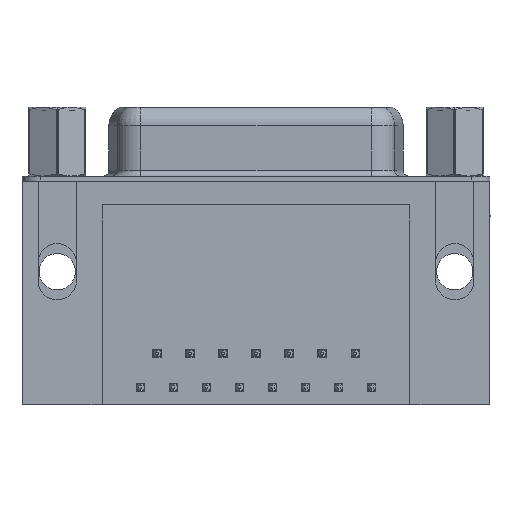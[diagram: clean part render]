
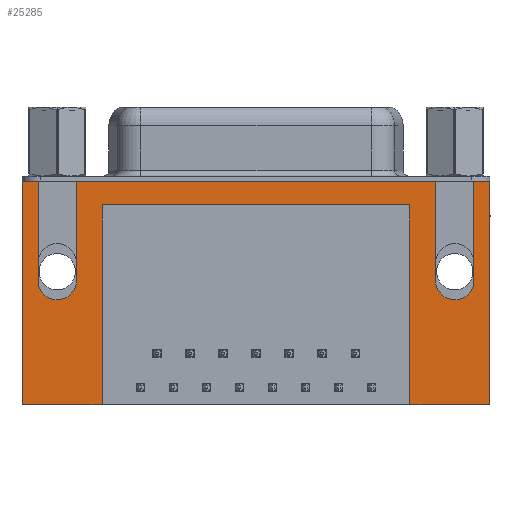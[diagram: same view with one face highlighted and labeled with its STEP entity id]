
A CAD part, front view. The second image highlights one B-rep face of the part: STEP entity #25285.
In plain terms, the highlighted planar face has unit normal (0, -1, 0).
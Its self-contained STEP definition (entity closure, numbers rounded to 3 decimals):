
#57 = EDGE_CURVE ( 'NONE', #28058, #2668, #22435, .T. ) ;
#464 = EDGE_CURVE ( 'NONE', #23235, #28058, #17280, .T. ) ;
#732 = FACE_OUTER_BOUND ( 'NONE', #28871, .T. ) ;
#1025 = EDGE_CURVE ( 'NONE', #8526, #19001, #14842, .T. ) ;
#1231 = DIRECTION ( 'NONE',  ( -1., 0., 0. ) ) ;
#1499 = LINE ( 'NONE', #9939, #1564 ) ;
#1564 = VECTOR ( 'NONE', #26962, 1000. ) ;
#1758 = CARTESIAN_POINT ( 'NONE',  ( 31.72, -6.275, 0. ) ) ;
#1853 = CARTESIAN_POINT ( 'NONE',  ( -2.935, -6.275, -2.5 ) ) ;
#2569 = VECTOR ( 'NONE', #21435, 1000. ) ;
#2662 = LINE ( 'NONE', #19008, #2569 ) ;
#2668 = VERTEX_POINT ( 'NONE', #8424 ) ;
#4235 = DIRECTION ( 'NONE',  ( 0., 0., 1. ) ) ;
#4272 = VERTEX_POINT ( 'NONE', #16402 ) ;
#4550 = DIRECTION ( 'NONE',  ( 0., 0., 1. ) ) ;
#4553 = VECTOR ( 'NONE', #14404, 1000. ) ;
#4650 = AXIS2_PLACEMENT_3D ( 'NONE', #19683, #5103, #22114 ) ;
#4806 = DIRECTION ( 'NONE',  ( 0., 0., -1. ) ) ;
#4980 = LINE ( 'NONE', #9600, #4553 ) ;
#5020 = ORIENTED_EDGE ( 'NONE', *, *, #29779, .F. ) ;
#5103 = DIRECTION ( 'NONE',  ( 0., -1., 0. ) ) ;
#5549 = VERTEX_POINT ( 'NONE', #13573 ) ;
#5914 = VERTEX_POINT ( 'NONE', #16620 ) ;
#6370 = CARTESIAN_POINT ( 'NONE',  ( 34.92, -6.275, 0. ) ) ;
#6408 = CARTESIAN_POINT ( 'NONE',  ( -2.935, -6.275, 0. ) ) ;
#6509 = DIRECTION ( 'NONE',  ( 0., -1., 0. ) ) ;
#6653 = CARTESIAN_POINT ( 'NONE',  ( -1.6, -6.275, 0. ) ) ;
#6703 = VERTEX_POINT ( 'NONE', #22931 ) ;
#6790 = ORIENTED_EDGE ( 'NONE', *, *, #464, .F. ) ;
#6910 = CARTESIAN_POINT ( 'NONE',  ( 36.255, -6.275, -18.76 ) ) ;
#7192 = VECTOR ( 'NONE', #26026, 1000. ) ;
#7223 = ORIENTED_EDGE ( 'NONE', *, *, #26447, .F. ) ;
#7283 = ORIENTED_EDGE ( 'NONE', *, *, #20444, .F. ) ;
#7373 = EDGE_CURVE ( 'NONE', #11342, #30143, #14511, .T. ) ;
#7556 = LINE ( 'NONE', #6408, #7192 ) ;
#8424 = CARTESIAN_POINT ( 'NONE',  ( 29.555, -6.275, -2. ) ) ;
#8526 = VERTEX_POINT ( 'NONE', #12347 ) ;
#8750 = CARTESIAN_POINT ( 'NONE',  ( 34.92, -6.275, 0. ) ) ;
#8834 = EDGE_CURVE ( 'NONE', #17516, #10612, #7556, .T. ) ;
#9586 = CARTESIAN_POINT ( 'NONE',  ( 36.255, -6.275, 0. ) ) ;
#9600 = CARTESIAN_POINT ( 'NONE',  ( 36.255, -6.275, -18.76 ) ) ;
#9855 = VECTOR ( 'NONE', #26143, 1000. ) ;
#9884 = LINE ( 'NONE', #6653, #9855 ) ;
#9939 = CARTESIAN_POINT ( 'NONE',  ( 31.72, -6.275, 0. ) ) ;
#10142 = EDGE_CURVE ( 'NONE', #19001, #5549, #1499, .T. ) ;
#10612 = VERTEX_POINT ( 'NONE', #9586 ) ;
#10784 = AXIS2_PLACEMENT_3D ( 'NONE', #24204, #19395, #4806 ) ;
#10906 = LINE ( 'NONE', #6370, #10937 ) ;
#10937 = VECTOR ( 'NONE', #23394, 1000. ) ;
#10995 = CARTESIAN_POINT ( 'NONE',  ( 3.765, -6.275, -2. ) ) ;
#11342 = VERTEX_POINT ( 'NONE', #25682 ) ;
#11384 = DIRECTION ( 'NONE',  ( -1., 0., 0. ) ) ;
#12347 = CARTESIAN_POINT ( 'NONE',  ( 1.6, -6.275, 0. ) ) ;
#12406 = EDGE_CURVE ( 'NONE', #6703, #24073, #23464, .T. ) ;
#13284 = DIRECTION ( 'NONE',  ( 1., 0., 0. ) ) ;
#13573 = CARTESIAN_POINT ( 'NONE',  ( 31.72, -6.275, -8.35 ) ) ;
#14277 = VECTOR ( 'NONE', #13284, 1000. ) ;
#14365 = ORIENTED_EDGE ( 'NONE', *, *, #24618, .T. ) ;
#14404 = DIRECTION ( 'NONE',  ( -1., 0., 0. ) ) ;
#14511 = CIRCLE ( 'NONE', #26122, 1.6 ) ;
#14842 = LINE ( 'NONE', #17664, #14927 ) ;
#14927 = VECTOR ( 'NONE', #28921, 1000. ) ;
#14974 = LINE ( 'NONE', #15721, #14277 ) ;
#15721 = CARTESIAN_POINT ( 'NONE',  ( -2.935, -6.275, 0. ) ) ;
#16050 = EDGE_CURVE ( 'NONE', #2668, #6703, #30447, .T. ) ;
#16227 = CARTESIAN_POINT ( 'NONE',  ( 29.555, -6.275, -2. ) ) ;
#16236 = ORIENTED_EDGE ( 'NONE', *, *, #18652, .F. ) ;
#16402 = CARTESIAN_POINT ( 'NONE',  ( -1.6, -6.275, 0. ) ) ;
#16620 = CARTESIAN_POINT ( 'NONE',  ( -2.935, -6.275, -18.76 ) ) ;
#16688 = VERTEX_POINT ( 'NONE', #18237 ) ;
#16695 = ORIENTED_EDGE ( 'NONE', *, *, #19280, .F. ) ;
#16969 = PLANE ( 'NONE',  #10784 ) ;
#17258 = CARTESIAN_POINT ( 'NONE',  ( 1.6, -6.275, -8.35 ) ) ;
#17280 = LINE ( 'NONE', #6910, #17444 ) ;
#17444 = VECTOR ( 'NONE', #11384, 1000. ) ;
#17516 = VERTEX_POINT ( 'NONE', #8750 ) ;
#17664 = CARTESIAN_POINT ( 'NONE',  ( -2.935, -6.275, 0. ) ) ;
#17811 = ORIENTED_EDGE ( 'NONE', *, *, #7373, .F. ) ;
#18237 = CARTESIAN_POINT ( 'NONE',  ( 34.92, -6.275, -8.35 ) ) ;
#18249 = ORIENTED_EDGE ( 'NONE', *, *, #1025, .F. ) ;
#18387 = DIRECTION ( 'NONE',  ( 0., 0., -1. ) ) ;
#18415 = CIRCLE ( 'NONE', #4650, 1.6 ) ;
#18580 = CARTESIAN_POINT ( 'NONE',  ( 36.255, -6.275, -18.76 ) ) ;
#18652 = EDGE_CURVE ( 'NONE', #5914, #19382, #20397, .T. ) ;
#18719 = ORIENTED_EDGE ( 'NONE', *, *, #21920, .F. ) ;
#19001 = VERTEX_POINT ( 'NONE', #1758 ) ;
#19008 = CARTESIAN_POINT ( 'NONE',  ( 36.255, -6.275, -2.5 ) ) ;
#19148 = DIRECTION ( 'NONE',  ( 0., 0., 1. ) ) ;
#19280 = EDGE_CURVE ( 'NONE', #5549, #16688, #18415, .T. ) ;
#19382 = VERTEX_POINT ( 'NONE', #20629 ) ;
#19395 = DIRECTION ( 'NONE',  ( 0., -1., 0. ) ) ;
#19683 = CARTESIAN_POINT ( 'NONE',  ( 33.32, -6.275, -8.35 ) ) ;
#20329 = VECTOR ( 'NONE', #4235, 1000. ) ;
#20397 = LINE ( 'NONE', #1853, #20329 ) ;
#20444 = EDGE_CURVE ( 'NONE', #19382, #4272, #14974, .T. ) ;
#20629 = CARTESIAN_POINT ( 'NONE',  ( -2.935, -6.275, 0. ) ) ;
#20729 = ORIENTED_EDGE ( 'NONE', *, *, #27681, .F. ) ;
#20823 = CARTESIAN_POINT ( 'NONE',  ( 3.765, -6.275, -2. ) ) ;
#21048 = CARTESIAN_POINT ( 'NONE',  ( 0., -6.275, -8.35 ) ) ;
#21435 = DIRECTION ( 'NONE',  ( 0., 0., 1. ) ) ;
#21566 = CARTESIAN_POINT ( 'NONE',  ( 1.6, -6.275, 0. ) ) ;
#21920 = EDGE_CURVE ( 'NONE', #4272, #11342, #9884, .T. ) ;
#22114 = DIRECTION ( 'NONE',  ( -1., 0., 0. ) ) ;
#22176 = VECTOR ( 'NONE', #19148, 1000. ) ;
#22435 = LINE ( 'NONE', #16227, #22176 ) ;
#22582 = ORIENTED_EDGE ( 'NONE', *, *, #57, .F. ) ;
#22705 = ORIENTED_EDGE ( 'NONE', *, *, #10142, .F. ) ;
#22788 = CARTESIAN_POINT ( 'NONE',  ( 3.765, -6.275, -18.76 ) ) ;
#22931 = CARTESIAN_POINT ( 'NONE',  ( 3.765, -6.275, -2. ) ) ;
#23192 = VECTOR ( 'NONE', #18387, 1000. ) ;
#23235 = VERTEX_POINT ( 'NONE', #18580 ) ;
#23394 = DIRECTION ( 'NONE',  ( 0., 0., 1. ) ) ;
#23464 = LINE ( 'NONE', #20823, #23192 ) ;
#23470 = CARTESIAN_POINT ( 'NONE',  ( 29.555, -6.275, -18.76 ) ) ;
#23515 = DIRECTION ( 'NONE',  ( 1., 0., 0. ) ) ;
#23911 = ORIENTED_EDGE ( 'NONE', *, *, #8834, .F. ) ;
#24073 = VERTEX_POINT ( 'NONE', #22788 ) ;
#24204 = CARTESIAN_POINT ( 'NONE',  ( -2.935, -6.275, -2.5 ) ) ;
#24616 = VECTOR ( 'NONE', #4550, 1000. ) ;
#24618 = EDGE_CURVE ( 'NONE', #23235, #10612, #2662, .T. ) ;
#24680 = LINE ( 'NONE', #21566, #24616 ) ;
#25285 = ADVANCED_FACE ( 'NONE', ( #732 ), #16969, .T. ) ;
#25682 = CARTESIAN_POINT ( 'NONE',  ( -1.6, -6.275, -8.35 ) ) ;
#26026 = DIRECTION ( 'NONE',  ( 1., 0., 0. ) ) ;
#26122 = AXIS2_PLACEMENT_3D ( 'NONE', #21048, #6509, #23515 ) ;
#26143 = DIRECTION ( 'NONE',  ( 0., 0., -1. ) ) ;
#26447 = EDGE_CURVE ( 'NONE', #24073, #5914, #4980, .T. ) ;
#26962 = DIRECTION ( 'NONE',  ( 0., 0., -1. ) ) ;
#27681 = EDGE_CURVE ( 'NONE', #30143, #8526, #24680, .T. ) ;
#27783 = ORIENTED_EDGE ( 'NONE', *, *, #16050, .F. ) ;
#28058 = VERTEX_POINT ( 'NONE', #23470 ) ;
#28871 = EDGE_LOOP ( 'NONE', ( #5020, #16695, #22705, #18249, #20729, #17811, #18719, #7283, #16236, #7223, #29409, #27783, #22582, #6790, #14365, #23911 ) ) ;
#28921 = DIRECTION ( 'NONE',  ( 1., 0., 0. ) ) ;
#29409 = ORIENTED_EDGE ( 'NONE', *, *, #12406, .F. ) ;
#29779 = EDGE_CURVE ( 'NONE', #16688, #17516, #10906, .T. ) ;
#30143 = VERTEX_POINT ( 'NONE', #17258 ) ;
#30361 = VECTOR ( 'NONE', #1231, 1000. ) ;
#30447 = LINE ( 'NONE', #10995, #30361 ) ;
